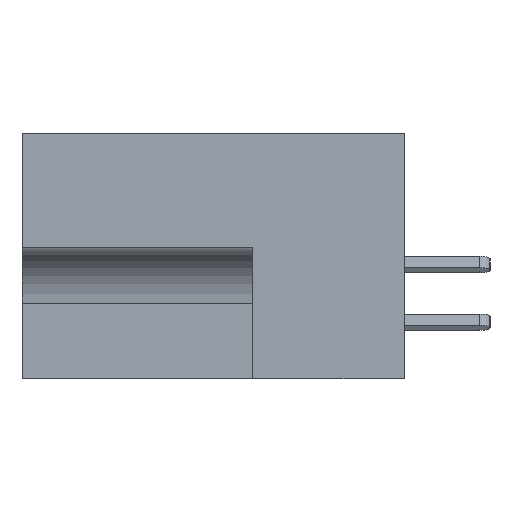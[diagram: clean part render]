
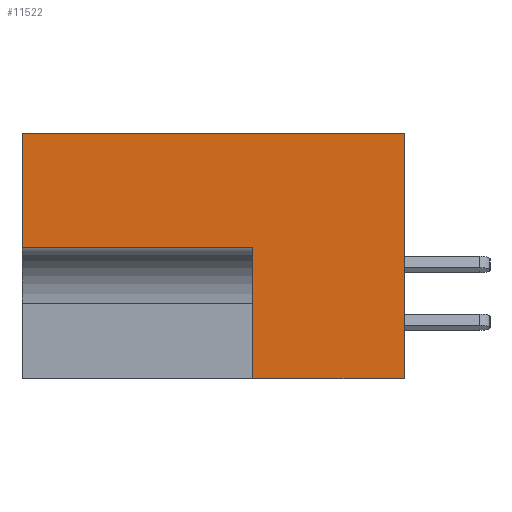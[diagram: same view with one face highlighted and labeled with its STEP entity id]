
A CAD part, left-side view. The second image highlights one B-rep face of the part: STEP entity #11522.
In plain terms, the highlighted planar face has unit normal (-1, 0, 0).
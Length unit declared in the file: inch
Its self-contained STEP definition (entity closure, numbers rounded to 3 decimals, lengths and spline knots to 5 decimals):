
#402 = VECTOR ( 'NONE', #11731, 39.37008 ) ;
#532 = EDGE_CURVE ( 'NONE', #9798, #9432, #1187, .T. ) ;
#1135 = DIRECTION ( 'NONE',  ( 0., 0., -1. ) ) ;
#1187 = LINE ( 'NONE', #10846, #6190 ) ;
#1321 = EDGE_CURVE ( 'NONE', #11377, #9798, #19279, .T. ) ;
#1407 = CARTESIAN_POINT ( 'NONE',  ( 0., 0.328, -0.531 ) ) ;
#1470 = ORIENTED_EDGE ( 'NONE', *, *, #14640, .F. ) ;
#3159 = ORIENTED_EDGE ( 'NONE', *, *, #532, .F. ) ;
#3249 = CARTESIAN_POINT ( 'NONE',  ( 0., 0.453, 0. ) ) ;
#3779 = LINE ( 'NONE', #8451, #15444 ) ;
#4218 = DIRECTION ( 'NONE',  ( 1., 0., 0. ) ) ;
#5823 = CARTESIAN_POINT ( 'NONE',  ( 0., 0., 0. ) ) ;
#6075 = VERTEX_POINT ( 'NONE', #10964 ) ;
#6190 = VECTOR ( 'NONE', #12378, 39.37008 ) ;
#7147 = ORIENTED_EDGE ( 'NONE', *, *, #10937, .T. ) ;
#7360 = DIRECTION ( 'NONE',  ( 0., 0., 1. ) ) ;
#7391 = EDGE_CURVE ( 'NONE', #9432, #18532, #13625, .T. ) ;
#7460 = VERTEX_POINT ( 'NONE', #5823 ) ;
#7638 = LINE ( 'NONE', #3249, #16026 ) ;
#8019 = EDGE_LOOP ( 'NONE', ( #18363, #3159, #14786, #11499, #7147, #1470 ) ) ;
#8029 = DIRECTION ( 'NONE',  ( 0., -1., 0. ) ) ;
#8230 = CARTESIAN_POINT ( 'NONE',  ( 0., 0.828, -0.248 ) ) ;
#8356 = CARTESIAN_POINT ( 'NONE',  ( 0., 0.328, -0.531 ) ) ;
#8451 = CARTESIAN_POINT ( 'NONE',  ( 0., 0., 0. ) ) ;
#8820 = CARTESIAN_POINT ( 'NONE',  ( 0., 0.828, 0. ) ) ;
#9432 = VERTEX_POINT ( 'NONE', #8230 ) ;
#9798 = VERTEX_POINT ( 'NONE', #12386 ) ;
#10846 = CARTESIAN_POINT ( 'NONE',  ( 0., 0.328, -0.248 ) ) ;
#10937 = EDGE_CURVE ( 'NONE', #6075, #7460, #3779, .T. ) ;
#10964 = CARTESIAN_POINT ( 'NONE',  ( 0., 0., -0.531 ) ) ;
#11377 = VERTEX_POINT ( 'NONE', #8356 ) ;
#11499 = ORIENTED_EDGE ( 'NONE', *, *, #11533, .T. ) ;
#11522 = ADVANCED_FACE ( 'NONE', ( #18287 ), #18082, .F. ) ;
#11533 = EDGE_CURVE ( 'NONE', #11377, #6075, #19236, .T. ) ;
#11731 = DIRECTION ( 'NONE',  ( 0., -1., 0. ) ) ;
#12378 = DIRECTION ( 'NONE',  ( 0., 1., 0. ) ) ;
#12386 = CARTESIAN_POINT ( 'NONE',  ( 0., 0.328, -0.248 ) ) ;
#13625 = LINE ( 'NONE', #8820, #18172 ) ;
#14329 = DIRECTION ( 'NONE',  ( 0., 0., 1. ) ) ;
#14640 = EDGE_CURVE ( 'NONE', #18532, #7460, #7638, .T. ) ;
#14786 = ORIENTED_EDGE ( 'NONE', *, *, #1321, .F. ) ;
#15444 = VECTOR ( 'NONE', #14329, 39.37008 ) ;
#15966 = VECTOR ( 'NONE', #16621, 39.37008 ) ;
#16026 = VECTOR ( 'NONE', #8029, 39.37008 ) ;
#16441 = AXIS2_PLACEMENT_3D ( 'NONE', #19598, #4218, #1135 ) ;
#16621 = DIRECTION ( 'NONE',  ( 0., 0., 1. ) ) ;
#18014 = CARTESIAN_POINT ( 'NONE',  ( 0., 0.453, -0.531 ) ) ;
#18082 = PLANE ( 'NONE',  #16441 ) ;
#18172 = VECTOR ( 'NONE', #7360, 39.37008 ) ;
#18287 = FACE_OUTER_BOUND ( 'NONE', #8019, .T. ) ;
#18363 = ORIENTED_EDGE ( 'NONE', *, *, #7391, .F. ) ;
#18532 = VERTEX_POINT ( 'NONE', #18755 ) ;
#18755 = CARTESIAN_POINT ( 'NONE',  ( 0., 0.828, 0. ) ) ;
#19236 = LINE ( 'NONE', #18014, #402 ) ;
#19279 = LINE ( 'NONE', #1407, #15966 ) ;
#19598 = CARTESIAN_POINT ( 'NONE',  ( 0., 0.453, 0. ) ) ;
